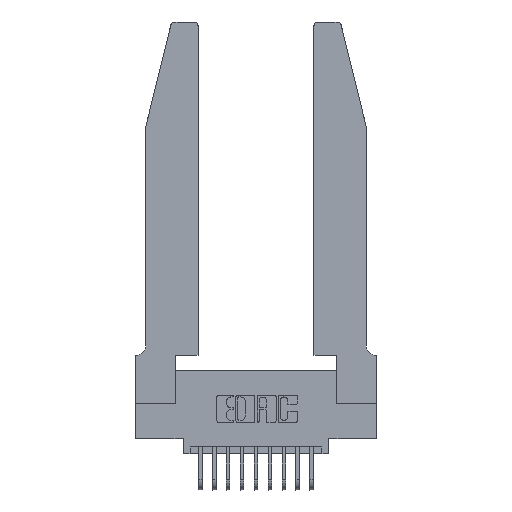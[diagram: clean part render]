
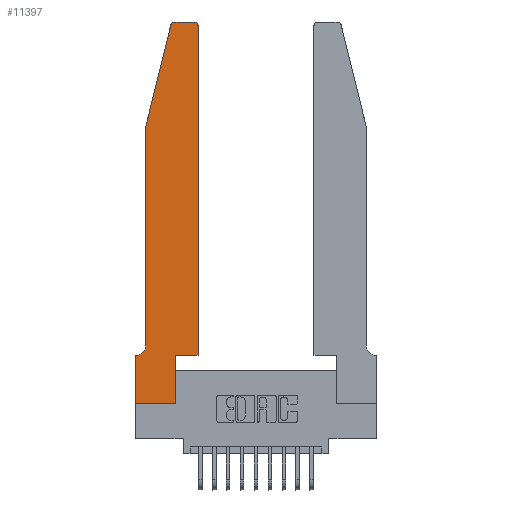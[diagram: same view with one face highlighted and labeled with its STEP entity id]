
A CAD part, top view. The second image highlights one B-rep face of the part: STEP entity #11397.
In plain terms, the highlighted planar face has unit normal (0, 0, 1).
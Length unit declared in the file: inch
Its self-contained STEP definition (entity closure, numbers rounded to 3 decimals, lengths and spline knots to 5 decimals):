
#185 = DIRECTION ( 'NONE',  ( -1., 0., 0. ) ) ;
#308 = DIRECTION ( 'NONE',  ( 1., 0., 0. ) ) ;
#319 = ORIENTED_EDGE ( 'NONE', *, *, #5095, .T. ) ;
#330 = DIRECTION ( 'NONE',  ( 0., 0., 1. ) ) ;
#350 = CARTESIAN_POINT ( 'NONE',  ( 0.4205, 2.72, 0.37 ) ) ;
#633 = VERTEX_POINT ( 'NONE', #5368 ) ;
#807 = VECTOR ( 'NONE', #17721, 39.37008 ) ;
#849 = LINE ( 'NONE', #5757, #12165 ) ;
#926 = VERTEX_POINT ( 'NONE', #15781 ) ;
#1023 = CARTESIAN_POINT ( 'NONE',  ( 0.0055, 0.35, 0.37 ) ) ;
#1306 = EDGE_CURVE ( 'NONE', #13626, #926, #5411, .T. ) ;
#1611 = DIRECTION ( 'NONE',  ( -0.239, -0.971, 0. ) ) ;
#1626 = LINE ( 'NONE', #15547, #16044 ) ;
#1999 = CIRCLE ( 'NONE', #6247, 0.03 ) ;
#2038 = VERTEX_POINT ( 'NONE', #5295 ) ;
#2534 = CARTESIAN_POINT ( 'NONE',  ( 0.0755, 0.42, 0.37 ) ) ;
#2783 = CARTESIAN_POINT ( 'NONE',  ( 0., 0., 0.37 ) ) ;
#2995 = CARTESIAN_POINT ( 'NONE',  ( 0.0755, 0.35, 0.37 ) ) ;
#3034 = ORIENTED_EDGE ( 'NONE', *, *, #10383, .T. ) ;
#3060 = DIRECTION ( 'NONE',  ( -1., 0., 0. ) ) ;
#3217 = ORIENTED_EDGE ( 'NONE', *, *, #16103, .T. ) ;
#4198 = ORIENTED_EDGE ( 'NONE', *, *, #17170, .T. ) ;
#4568 = CARTESIAN_POINT ( 'NONE',  ( 0., 0., 0.37 ) ) ;
#4880 = CARTESIAN_POINT ( 'NONE',  ( 0., 0.35, 0.37 ) ) ;
#5056 = ORIENTED_EDGE ( 'NONE', *, *, #6827, .T. ) ;
#5095 = EDGE_CURVE ( 'NONE', #8624, #7591, #1626, .T. ) ;
#5267 = VERTEX_POINT ( 'NONE', #15840 ) ;
#5295 = CARTESIAN_POINT ( 'NONE',  ( 0.4505, 0.35, 0.37 ) ) ;
#5368 = CARTESIAN_POINT ( 'NONE',  ( 0.284, 2.75, 0.37 ) ) ;
#5376 = VECTOR ( 'NONE', #9528, 39.37008 ) ;
#5392 = VECTOR ( 'NONE', #3060, 39.37008 ) ;
#5411 = CIRCLE ( 'NONE', #15062, 0.03 ) ;
#5449 = CARTESIAN_POINT ( 'NONE',  ( 0.4505, 0.35, 0.37 ) ) ;
#5613 = LINE ( 'NONE', #5449, #807 ) ;
#5619 = LINE ( 'NONE', #9721, #8916 ) ;
#5677 = DIRECTION ( 'NONE',  ( 0., -1., 0. ) ) ;
#5688 = EDGE_CURVE ( 'NONE', #17743, #11016, #12001, .T. ) ;
#5694 = LINE ( 'NONE', #10983, #16215 ) ;
#5757 = CARTESIAN_POINT ( 'NONE',  ( 0.2605, 2.75, 0.37 ) ) ;
#6047 = DIRECTION ( 'NONE',  ( 1., 0., 0. ) ) ;
#6066 = CARTESIAN_POINT ( 'NONE',  ( 0.284, 2.72, 0.37 ) ) ;
#6247 = AXIS2_PLACEMENT_3D ( 'NONE', #6066, #15677, #7520 ) ;
#6298 = DIRECTION ( 'NONE',  ( 1., 0., 0. ) ) ;
#6793 = AXIS2_PLACEMENT_3D ( 'NONE', #4880, #14544, #6298 ) ;
#6827 = EDGE_CURVE ( 'NONE', #5267, #14348, #7461, .T. ) ;
#6998 = VECTOR ( 'NONE', #5677, 39.37008 ) ;
#7102 = CARTESIAN_POINT ( 'NONE',  ( 0., 0., 0.37 ) ) ;
#7431 = CARTESIAN_POINT ( 'NONE',  ( 0.25487, 2.72718, 0.37 ) ) ;
#7461 = LINE ( 'NONE', #7102, #6998 ) ;
#7520 = DIRECTION ( 'NONE',  ( 1., 0., 0. ) ) ;
#7591 = VERTEX_POINT ( 'NONE', #12079 ) ;
#8108 = EDGE_LOOP ( 'NONE', ( #3217, #10612, #319, #3034, #10661, #4198, #5056, #15302, #13493, #10815, #13011, #17260 ) ) ;
#8145 = CARTESIAN_POINT ( 'NONE',  ( 0.2865, 0.35, 0.37 ) ) ;
#8624 = VERTEX_POINT ( 'NONE', #7431 ) ;
#8858 = DIRECTION ( 'NONE',  ( 0., 0., -1. ) ) ;
#8916 = VECTOR ( 'NONE', #11106, 39.37008 ) ;
#9111 = EDGE_CURVE ( 'NONE', #2038, #13626, #5613, .T. ) ;
#9528 = DIRECTION ( 'NONE',  ( 0., 1., 0. ) ) ;
#9721 = CARTESIAN_POINT ( 'NONE',  ( 0.4505, 0.35, 0.37 ) ) ;
#9830 = LINE ( 'NONE', #4568, #13023 ) ;
#10383 = EDGE_CURVE ( 'NONE', #7591, #17743, #5694, .T. ) ;
#10460 = PLANE ( 'NONE',  #6793 ) ;
#10612 = ORIENTED_EDGE ( 'NONE', *, *, #16246, .T. ) ;
#10661 = ORIENTED_EDGE ( 'NONE', *, *, #5688, .T. ) ;
#10815 = ORIENTED_EDGE ( 'NONE', *, *, #16969, .T. ) ;
#10847 = CARTESIAN_POINT ( 'NONE',  ( 0.4505, 2.72, 0.37 ) ) ;
#10983 = CARTESIAN_POINT ( 'NONE',  ( 0.0755, 2., 0.37 ) ) ;
#11016 = VERTEX_POINT ( 'NONE', #1023 ) ;
#11106 = DIRECTION ( 'NONE',  ( 1., 0., 0. ) ) ;
#11296 = EDGE_CURVE ( 'NONE', #14348, #12890, #9830, .T. ) ;
#11397 = ADVANCED_FACE ( 'NONE', ( #14941 ), #10460, .T. ) ;
#12001 = CIRCLE ( 'NONE', #12151, 0.07 ) ;
#12079 = CARTESIAN_POINT ( 'NONE',  ( 0.0755, 2., 0.37 ) ) ;
#12151 = AXIS2_PLACEMENT_3D ( 'NONE', #16950, #8858, #185 ) ;
#12165 = VECTOR ( 'NONE', #16713, 39.37008 ) ;
#12744 = LINE ( 'NONE', #8145, #5376 ) ;
#12890 = VERTEX_POINT ( 'NONE', #14523 ) ;
#13011 = ORIENTED_EDGE ( 'NONE', *, *, #9111, .T. ) ;
#13023 = VECTOR ( 'NONE', #6047, 39.37008 ) ;
#13332 = CARTESIAN_POINT ( 'NONE',  ( 0.2865, 0.35, 0.37 ) ) ;
#13493 = ORIENTED_EDGE ( 'NONE', *, *, #17665, .T. ) ;
#13541 = VERTEX_POINT ( 'NONE', #13332 ) ;
#13626 = VERTEX_POINT ( 'NONE', #10847 ) ;
#14348 = VERTEX_POINT ( 'NONE', #2783 ) ;
#14523 = CARTESIAN_POINT ( 'NONE',  ( 0.2865, 0., 0.37 ) ) ;
#14544 = DIRECTION ( 'NONE',  ( 0., 0., 1. ) ) ;
#14941 = FACE_OUTER_BOUND ( 'NONE', #8108, .T. ) ;
#15051 = DIRECTION ( 'NONE',  ( 0., -1., 0. ) ) ;
#15062 = AXIS2_PLACEMENT_3D ( 'NONE', #350, #330, #308 ) ;
#15302 = ORIENTED_EDGE ( 'NONE', *, *, #11296, .T. ) ;
#15547 = CARTESIAN_POINT ( 'NONE',  ( 0.0755, 2., 0.37 ) ) ;
#15677 = DIRECTION ( 'NONE',  ( 0., 0., 1. ) ) ;
#15781 = CARTESIAN_POINT ( 'NONE',  ( 0.4205, 2.75, 0.37 ) ) ;
#15840 = CARTESIAN_POINT ( 'NONE',  ( 0., 0.35, 0.37 ) ) ;
#16044 = VECTOR ( 'NONE', #1611, 39.37008 ) ;
#16103 = EDGE_CURVE ( 'NONE', #926, #633, #849, .T. ) ;
#16215 = VECTOR ( 'NONE', #15051, 39.37008 ) ;
#16246 = EDGE_CURVE ( 'NONE', #633, #8624, #1999, .T. ) ;
#16330 = LINE ( 'NONE', #2995, #5392 ) ;
#16713 = DIRECTION ( 'NONE',  ( -1., 0., 0. ) ) ;
#16950 = CARTESIAN_POINT ( 'NONE',  ( 0.0055, 0.42, 0.37 ) ) ;
#16969 = EDGE_CURVE ( 'NONE', #13541, #2038, #5619, .T. ) ;
#17170 = EDGE_CURVE ( 'NONE', #11016, #5267, #16330, .T. ) ;
#17260 = ORIENTED_EDGE ( 'NONE', *, *, #1306, .T. ) ;
#17665 = EDGE_CURVE ( 'NONE', #12890, #13541, #12744, .T. ) ;
#17721 = DIRECTION ( 'NONE',  ( 0., 1., 0. ) ) ;
#17743 = VERTEX_POINT ( 'NONE', #2534 ) ;
